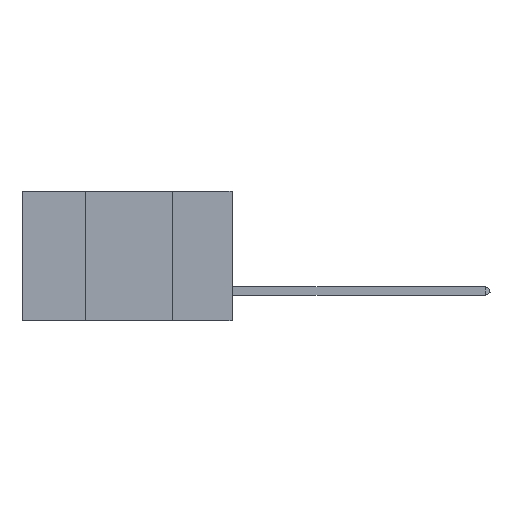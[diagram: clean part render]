
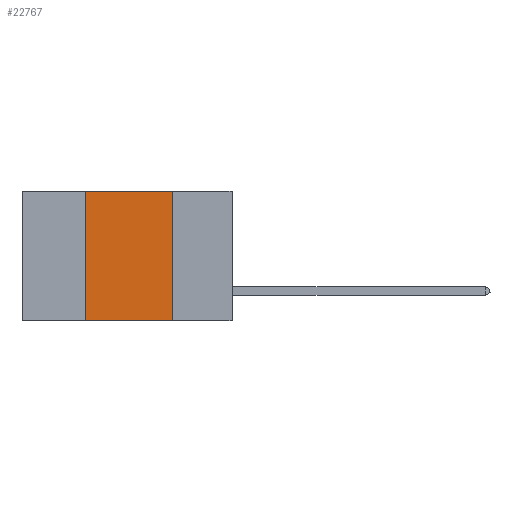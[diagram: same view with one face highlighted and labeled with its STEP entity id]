
A CAD part, left-side view. The second image highlights one B-rep face of the part: STEP entity #22767.
In plain terms, the highlighted planar face has unit normal (-1, 0, 0).
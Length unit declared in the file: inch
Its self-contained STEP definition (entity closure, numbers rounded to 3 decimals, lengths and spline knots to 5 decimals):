
#514 = VECTOR ( 'NONE', #40429, 39.37008 ) ;
#977 = LINE ( 'NONE', #4992, #14843 ) ;
#1659 = LINE ( 'NONE', #26090, #514 ) ;
#2210 = DIRECTION ( 'NONE',  ( 0., 0., -1. ) ) ;
#2421 = VECTOR ( 'NONE', #21425, 39.37008 ) ;
#4742 = EDGE_CURVE ( 'NONE', #6770, #41057, #19571, .T. ) ;
#4992 = CARTESIAN_POINT ( 'NONE',  ( 0., 0.6, -0.37 ) ) ;
#5091 = CARTESIAN_POINT ( 'NONE',  ( 0., 0.17, 0. ) ) ;
#5330 = EDGE_CURVE ( 'NONE', #18468, #39071, #21520, .T. ) ;
#6770 = VERTEX_POINT ( 'NONE', #5091 ) ;
#6982 = ORIENTED_EDGE ( 'NONE', *, *, #4742, .F. ) ;
#7960 = ORIENTED_EDGE ( 'NONE', *, *, #25738, .T. ) ;
#8542 = CARTESIAN_POINT ( 'NONE',  ( 0., 0.17, 0. ) ) ;
#8712 = ORIENTED_EDGE ( 'NONE', *, *, #5330, .F. ) ;
#14843 = VECTOR ( 'NONE', #32358, 39.37008 ) ;
#16046 = DIRECTION ( 'NONE',  ( 1., 0., 0. ) ) ;
#18468 = VERTEX_POINT ( 'NONE', #26078 ) ;
#19515 = PLANE ( 'NONE',  #36322 ) ;
#19571 = LINE ( 'NONE', #8542, #24210 ) ;
#21425 = DIRECTION ( 'NONE',  ( 0., 0., 1. ) ) ;
#21520 = LINE ( 'NONE', #38423, #2421 ) ;
#22767 = ADVANCED_FACE ( 'NONE', ( #23609 ), #19515, .F. ) ;
#23609 = FACE_OUTER_BOUND ( 'NONE', #31191, .T. ) ;
#24210 = VECTOR ( 'NONE', #35952, 39.37008 ) ;
#25738 = EDGE_CURVE ( 'NONE', #18468, #41057, #977, .T. ) ;
#26078 = CARTESIAN_POINT ( 'NONE',  ( 0., 0.42, -0.37 ) ) ;
#26090 = CARTESIAN_POINT ( 'NONE',  ( 0., 0.6, 0. ) ) ;
#26959 = CARTESIAN_POINT ( 'NONE',  ( 0., 0.42, 0. ) ) ;
#31191 = EDGE_LOOP ( 'NONE', ( #6982, #37748, #8712, #7960 ) ) ;
#32358 = DIRECTION ( 'NONE',  ( 0., -1., 0. ) ) ;
#35952 = DIRECTION ( 'NONE',  ( 0., 0., -1. ) ) ;
#36322 = AXIS2_PLACEMENT_3D ( 'NONE', #40190, #16046, #2210 ) ;
#37748 = ORIENTED_EDGE ( 'NONE', *, *, #43707, .F. ) ;
#38423 = CARTESIAN_POINT ( 'NONE',  ( 0., 0.42, 0. ) ) ;
#39071 = VERTEX_POINT ( 'NONE', #26959 ) ;
#40190 = CARTESIAN_POINT ( 'NONE',  ( 0., 0.6, 0. ) ) ;
#40429 = DIRECTION ( 'NONE',  ( 0., -1., 0. ) ) ;
#41057 = VERTEX_POINT ( 'NONE', #41833 ) ;
#41833 = CARTESIAN_POINT ( 'NONE',  ( 0., 0.17, -0.37 ) ) ;
#43707 = EDGE_CURVE ( 'NONE', #39071, #6770, #1659, .T. ) ;
